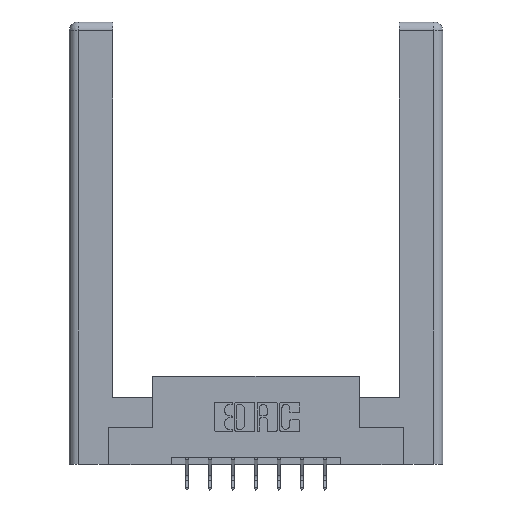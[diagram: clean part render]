
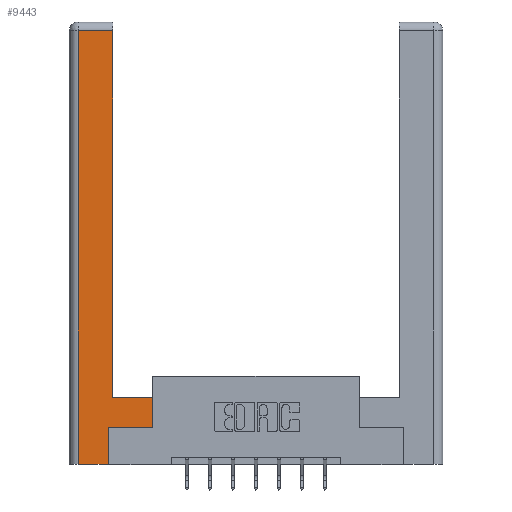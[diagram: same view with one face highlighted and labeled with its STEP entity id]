
A CAD part, top view. The second image highlights one B-rep face of the part: STEP entity #9443.
In plain terms, the highlighted planar face has unit normal (0, 0, 1).
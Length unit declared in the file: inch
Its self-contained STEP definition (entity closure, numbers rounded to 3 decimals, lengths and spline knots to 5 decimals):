
#8 = LINE ( 'NONE', #4751, #9774 ) ;
#167 = DIRECTION ( 'NONE',  ( 0., 0., -1. ) ) ;
#511 = ORIENTED_EDGE ( 'NONE', *, *, #12670, .T. ) ;
#565 = EDGE_CURVE ( 'NONE', #10174, #2170, #8, .T. ) ;
#712 = EDGE_CURVE ( 'NONE', #9732, #10078, #2797, .T. ) ;
#743 = CARTESIAN_POINT ( 'NONE',  ( 0.565, 0.45, 0. ) ) ;
#1002 = FACE_OUTER_BOUND ( 'NONE', #11973, .T. ) ;
#1296 = DIRECTION ( 'NONE',  ( 1., 0., 0. ) ) ;
#1465 = VECTOR ( 'NONE', #8381, 39.37008 ) ;
#1614 = VERTEX_POINT ( 'NONE', #11556 ) ;
#2170 = VERTEX_POINT ( 'NONE', #12035 ) ;
#2761 = EDGE_CURVE ( 'NONE', #2170, #6386, #3672, .T. ) ;
#2790 = CARTESIAN_POINT ( 'NONE',  ( 0.0615, 2.94, 0. ) ) ;
#2797 = LINE ( 'NONE', #7051, #9933 ) ;
#3235 = ORIENTED_EDGE ( 'NONE', *, *, #712, .T. ) ;
#3318 = DIRECTION ( 'NONE',  ( 0., 1., 0. ) ) ;
#3479 = AXIS2_PLACEMENT_3D ( 'NONE', #12051, #167, #7299 ) ;
#3490 = LINE ( 'NONE', #12220, #10790 ) ;
#3595 = CARTESIAN_POINT ( 'NONE',  ( 0.565, 0.245, 0. ) ) ;
#3672 = LINE ( 'NONE', #11877, #4431 ) ;
#3945 = DIRECTION ( 'NONE',  ( 0., -1., 0. ) ) ;
#4431 = VECTOR ( 'NONE', #6784, 39.37008 ) ;
#4446 = CARTESIAN_POINT ( 'NONE',  ( 0.295, 2.94, 0. ) ) ;
#4588 = ORIENTED_EDGE ( 'NONE', *, *, #7663, .T. ) ;
#4751 = CARTESIAN_POINT ( 'NONE',  ( 0.295, 0.45, 0. ) ) ;
#5080 = PLANE ( 'NONE',  #3479 ) ;
#5526 = EDGE_CURVE ( 'NONE', #6452, #9732, #8018, .T. ) ;
#6243 = EDGE_CURVE ( 'NONE', #1614, #6452, #3490, .T. ) ;
#6386 = VERTEX_POINT ( 'NONE', #4446 ) ;
#6452 = VERTEX_POINT ( 'NONE', #8550 ) ;
#6784 = DIRECTION ( 'NONE',  ( 0., 1., 0. ) ) ;
#6933 = CARTESIAN_POINT ( 'NONE',  ( 0.0615, 0., 0. ) ) ;
#7051 = CARTESIAN_POINT ( 'NONE',  ( 0.565, 0.245, 0. ) ) ;
#7299 = DIRECTION ( 'NONE',  ( -1., 0., 0. ) ) ;
#7513 = ORIENTED_EDGE ( 'NONE', *, *, #6243, .T. ) ;
#7558 = VECTOR ( 'NONE', #9674, 39.37008 ) ;
#7603 = CARTESIAN_POINT ( 'NONE',  ( 0.265, 0.245, 0. ) ) ;
#7663 = EDGE_CURVE ( 'NONE', #7678, #1614, #11906, .T. ) ;
#7678 = VERTEX_POINT ( 'NONE', #2790 ) ;
#8018 = LINE ( 'NONE', #11639, #7558 ) ;
#8295 = CARTESIAN_POINT ( 'NONE',  ( 0.0615, 2.94, 0. ) ) ;
#8381 = DIRECTION ( 'NONE',  ( -1., 0., 0. ) ) ;
#8550 = CARTESIAN_POINT ( 'NONE',  ( 0.265, 0., 0. ) ) ;
#8624 = LINE ( 'NONE', #8295, #1465 ) ;
#9187 = ORIENTED_EDGE ( 'NONE', *, *, #2761, .T. ) ;
#9443 = ADVANCED_FACE ( 'NONE', ( #1002 ), #5080, .F. ) ;
#9674 = DIRECTION ( 'NONE',  ( 0., 1., 0. ) ) ;
#9732 = VERTEX_POINT ( 'NONE', #7603 ) ;
#9774 = VECTOR ( 'NONE', #9800, 39.37008 ) ;
#9800 = DIRECTION ( 'NONE',  ( -1., 0., 0. ) ) ;
#9933 = VECTOR ( 'NONE', #1296, 39.37008 ) ;
#10078 = VERTEX_POINT ( 'NONE', #3595 ) ;
#10174 = VERTEX_POINT ( 'NONE', #743 ) ;
#10666 = VECTOR ( 'NONE', #3945, 39.37008 ) ;
#10790 = VECTOR ( 'NONE', #12386, 39.37008 ) ;
#11303 = CARTESIAN_POINT ( 'NONE',  ( 0.565, 0.45, 0. ) ) ;
#11556 = CARTESIAN_POINT ( 'NONE',  ( 0.0615, 0., 0. ) ) ;
#11639 = CARTESIAN_POINT ( 'NONE',  ( 0.265, 0.245, 0. ) ) ;
#11831 = EDGE_CURVE ( 'NONE', #6386, #7678, #8624, .T. ) ;
#11840 = LINE ( 'NONE', #11303, #12762 ) ;
#11877 = CARTESIAN_POINT ( 'NONE',  ( 0.295, 3., 0. ) ) ;
#11906 = LINE ( 'NONE', #6933, #10666 ) ;
#11973 = EDGE_LOOP ( 'NONE', ( #9187, #12566, #4588, #7513, #12413, #3235, #511, #12463 ) ) ;
#12035 = CARTESIAN_POINT ( 'NONE',  ( 0.295, 0.45, 0. ) ) ;
#12051 = CARTESIAN_POINT ( 'NONE',  ( 0., 0., 0. ) ) ;
#12220 = CARTESIAN_POINT ( 'NONE',  ( 0.265, 0., 0. ) ) ;
#12386 = DIRECTION ( 'NONE',  ( 1., 0., 0. ) ) ;
#12413 = ORIENTED_EDGE ( 'NONE', *, *, #5526, .T. ) ;
#12463 = ORIENTED_EDGE ( 'NONE', *, *, #565, .T. ) ;
#12566 = ORIENTED_EDGE ( 'NONE', *, *, #11831, .T. ) ;
#12670 = EDGE_CURVE ( 'NONE', #10078, #10174, #11840, .T. ) ;
#12762 = VECTOR ( 'NONE', #3318, 39.37008 ) ;
